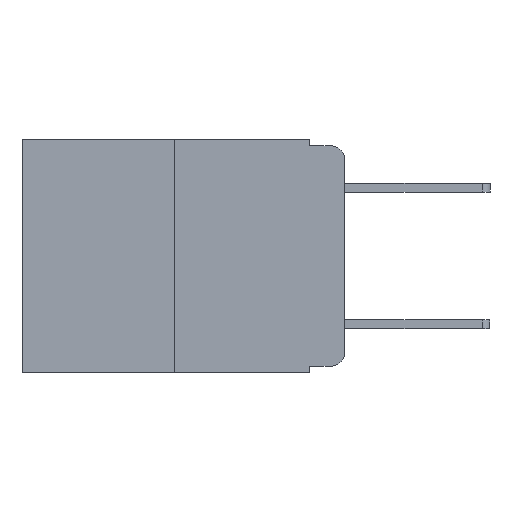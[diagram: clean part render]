
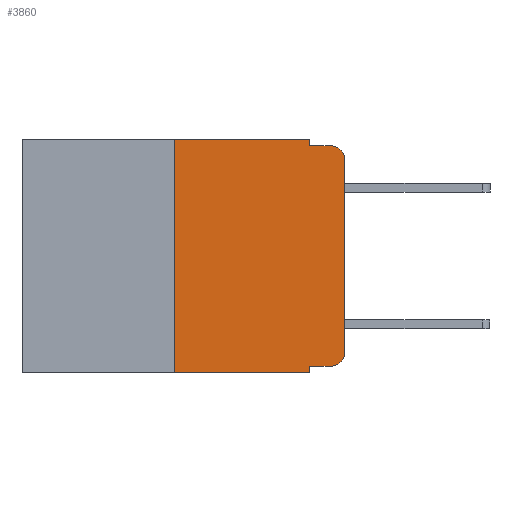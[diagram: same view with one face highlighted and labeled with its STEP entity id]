
A CAD part, left-side view. The second image highlights one B-rep face of the part: STEP entity #3860.
In plain terms, the highlighted planar face has unit normal (-1, 0, 0).
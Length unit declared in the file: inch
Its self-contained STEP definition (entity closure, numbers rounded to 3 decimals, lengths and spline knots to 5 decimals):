
#1 = EDGE_CURVE ( 'NONE', #15052, #5514, #4440, .T. ) ;
#9 = VERTEX_POINT ( 'NONE', #8927 ) ;
#215 = CARTESIAN_POINT ( 'NONE',  ( 0., 0.473, 0. ) ) ;
#285 = PLANE ( 'NONE',  #1481 ) ;
#339 = EDGE_CURVE ( 'NONE', #11672, #15052, #8793, .T. ) ;
#534 = EDGE_CURVE ( 'NONE', #14535, #5895, #9834, .T. ) ;
#749 = CARTESIAN_POINT ( 'NONE',  ( 0., 0.473, -0.343 ) ) ;
#772 = LINE ( 'NONE', #749, #9757 ) ;
#913 = VECTOR ( 'NONE', #5478, 39.37008 ) ;
#1309 = EDGE_CURVE ( 'NONE', #13584, #2826, #8426, .T. ) ;
#1314 = EDGE_CURVE ( 'NONE', #13584, #9, #4995, .T. ) ;
#1338 = EDGE_CURVE ( 'NONE', #9, #11463, #4585, .T. ) ;
#1481 = AXIS2_PLACEMENT_3D ( 'NONE', #215, #8970, #1682 ) ;
#1488 = EDGE_CURVE ( 'NONE', #14076, #5514, #9468, .T. ) ;
#1489 = VECTOR ( 'NONE', #6043, 39.37008 ) ;
#1682 = DIRECTION ( 'NONE',  ( 0., 0., -1. ) ) ;
#1903 = LINE ( 'NONE', #13645, #1489 ) ;
#1955 = VECTOR ( 'NONE', #8708, 39.37008 ) ;
#2080 = CARTESIAN_POINT ( 'NONE',  ( 0., 0.25, -0.343 ) ) ;
#2141 = DIRECTION ( 'NONE',  ( 0., 0., 1. ) ) ;
#2196 = ORIENTED_EDGE ( 'NONE', *, *, #339, .F. ) ;
#2388 = EDGE_CURVE ( 'NONE', #11463, #14076, #1903, .T. ) ;
#2715 = CARTESIAN_POINT ( 'NONE',  ( 0., 0.051, 0. ) ) ;
#2826 = VERTEX_POINT ( 'NONE', #11532 ) ;
#2909 = CARTESIAN_POINT ( 'NONE',  ( 0., 0.051, -0.01 ) ) ;
#3737 = CARTESIAN_POINT ( 'NONE',  ( 0., 0.051, -0.333 ) ) ;
#3860 = ADVANCED_FACE ( 'NONE', ( #5229 ), #285, .F. ) ;
#4440 = LINE ( 'NONE', #2909, #913 ) ;
#4582 = EDGE_CURVE ( 'NONE', #5895, #11672, #10657, .T. ) ;
#4585 = CIRCLE ( 'NONE', #14884, 0.02 ) ;
#4619 = CARTESIAN_POINT ( 'NONE',  ( 0., 0.051, 0. ) ) ;
#4725 = DIRECTION ( 'NONE',  ( -1., 0., 0. ) ) ;
#4995 = LINE ( 'NONE', #8147, #10665 ) ;
#5203 = CARTESIAN_POINT ( 'NONE',  ( 0., 0.051, 0. ) ) ;
#5229 = FACE_OUTER_BOUND ( 'NONE', #10812, .T. ) ;
#5235 = CARTESIAN_POINT ( 'NONE',  ( 0., 0.02, -0.03 ) ) ;
#5478 = DIRECTION ( 'NONE',  ( 0., -1., 0. ) ) ;
#5508 = CARTESIAN_POINT ( 'NONE',  ( 0., 0.02, -0.01 ) ) ;
#5514 = VERTEX_POINT ( 'NONE', #5508 ) ;
#5814 = CARTESIAN_POINT ( 'NONE',  ( 0., 0., -0.313 ) ) ;
#5845 = DIRECTION ( 'NONE',  ( 0., 0., -1. ) ) ;
#5895 = VERTEX_POINT ( 'NONE', #9621 ) ;
#6043 = DIRECTION ( 'NONE',  ( 0., 0., 1. ) ) ;
#6349 = ORIENTED_EDGE ( 'NONE', *, *, #1309, .F. ) ;
#6395 = DIRECTION ( 'NONE',  ( 0., 0., -1. ) ) ;
#6486 = CARTESIAN_POINT ( 'NONE',  ( 0., 0.051, -0.01 ) ) ;
#7124 = DIRECTION ( 'NONE',  ( 0., -1., 0. ) ) ;
#7945 = ORIENTED_EDGE ( 'NONE', *, *, #2388, .T. ) ;
#8066 = VECTOR ( 'NONE', #5845, 39.37008 ) ;
#8147 = CARTESIAN_POINT ( 'NONE',  ( 0., 0.051, -0.333 ) ) ;
#8168 = AXIS2_PLACEMENT_3D ( 'NONE', #5235, #12952, #6395 ) ;
#8308 = ORIENTED_EDGE ( 'NONE', *, *, #1488, .T. ) ;
#8426 = LINE ( 'NONE', #4619, #8066 ) ;
#8647 = ORIENTED_EDGE ( 'NONE', *, *, #4582, .F. ) ;
#8708 = DIRECTION ( 'NONE',  ( 0., 0., -1. ) ) ;
#8793 = LINE ( 'NONE', #2715, #1955 ) ;
#8835 = CARTESIAN_POINT ( 'NONE',  ( 0., 0.473, 0. ) ) ;
#8880 = DIRECTION ( 'NONE',  ( 0., -1., 0. ) ) ;
#8927 = CARTESIAN_POINT ( 'NONE',  ( 0., 0.02, -0.333 ) ) ;
#8970 = DIRECTION ( 'NONE',  ( 1., 0., 0. ) ) ;
#9267 = DIRECTION ( 'NONE',  ( 0., -1., 0. ) ) ;
#9353 = CARTESIAN_POINT ( 'NONE',  ( 0., 0.25, 0. ) ) ;
#9468 = CIRCLE ( 'NONE', #8168, 0.02 ) ;
#9621 = CARTESIAN_POINT ( 'NONE',  ( 0., 0.25, 0. ) ) ;
#9757 = VECTOR ( 'NONE', #7124, 39.37008 ) ;
#9834 = LINE ( 'NONE', #9353, #12671 ) ;
#10048 = ORIENTED_EDGE ( 'NONE', *, *, #1338, .T. ) ;
#10657 = LINE ( 'NONE', #8835, #13132 ) ;
#10665 = VECTOR ( 'NONE', #9267, 39.37008 ) ;
#10812 = EDGE_LOOP ( 'NONE', ( #7945, #8308, #14005, #2196, #8647, #11560, #14671, #6349, #12196, #10048 ) ) ;
#10986 = CARTESIAN_POINT ( 'NONE',  ( 0., 0., -0.03 ) ) ;
#11463 = VERTEX_POINT ( 'NONE', #5814 ) ;
#11504 = CARTESIAN_POINT ( 'NONE',  ( 0., 0.02, -0.313 ) ) ;
#11518 = EDGE_CURVE ( 'NONE', #14535, #2826, #772, .T. ) ;
#11532 = CARTESIAN_POINT ( 'NONE',  ( 0., 0.051, -0.343 ) ) ;
#11560 = ORIENTED_EDGE ( 'NONE', *, *, #534, .F. ) ;
#11672 = VERTEX_POINT ( 'NONE', #5203 ) ;
#12196 = ORIENTED_EDGE ( 'NONE', *, *, #1314, .T. ) ;
#12558 = DIRECTION ( 'NONE',  ( 0., 0., -1. ) ) ;
#12671 = VECTOR ( 'NONE', #2141, 39.37008 ) ;
#12952 = DIRECTION ( 'NONE',  ( -1., 0., 0. ) ) ;
#13132 = VECTOR ( 'NONE', #8880, 39.37008 ) ;
#13584 = VERTEX_POINT ( 'NONE', #3737 ) ;
#13645 = CARTESIAN_POINT ( 'NONE',  ( 0., 0., 0. ) ) ;
#14005 = ORIENTED_EDGE ( 'NONE', *, *, #1, .F. ) ;
#14076 = VERTEX_POINT ( 'NONE', #10986 ) ;
#14535 = VERTEX_POINT ( 'NONE', #2080 ) ;
#14671 = ORIENTED_EDGE ( 'NONE', *, *, #11518, .T. ) ;
#14884 = AXIS2_PLACEMENT_3D ( 'NONE', #11504, #4725, #12558 ) ;
#15052 = VERTEX_POINT ( 'NONE', #6486 ) ;
